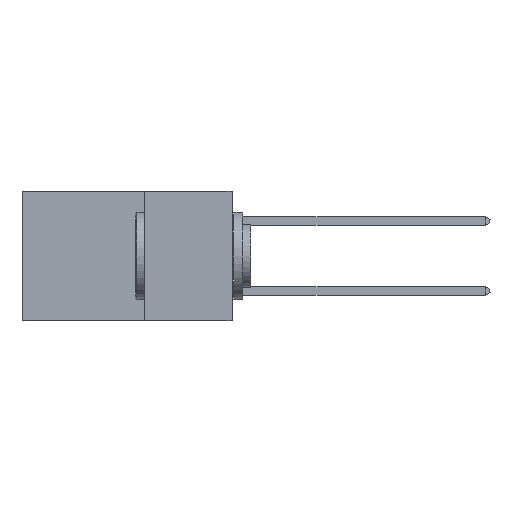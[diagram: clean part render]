
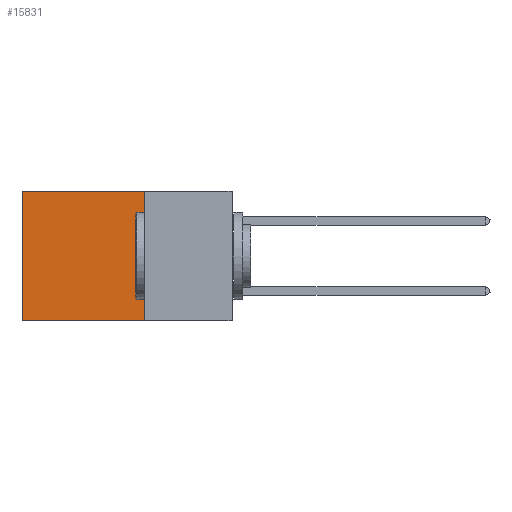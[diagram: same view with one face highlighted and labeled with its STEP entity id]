
A CAD part, left-side view. The second image highlights one B-rep face of the part: STEP entity #15831.
In plain terms, the highlighted planar face has unit normal (-1, 0, 0).
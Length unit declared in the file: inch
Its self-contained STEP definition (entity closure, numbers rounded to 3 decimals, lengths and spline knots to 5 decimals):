
#221 = EDGE_LOOP ( 'NONE', ( #6509, #34682, #23838, #32155 ) ) ;
#659 = VECTOR ( 'NONE', #8552, 39.37008 ) ;
#698 = EDGE_CURVE ( 'NONE', #30592, #21738, #38104, .T. ) ;
#722 = VECTOR ( 'NONE', #20256, 39.37008 ) ;
#741 = VERTEX_POINT ( 'NONE', #23607 ) ;
#1066 = VECTOR ( 'NONE', #27200, 39.37008 ) ;
#3652 = DIRECTION ( 'NONE',  ( 1., 0., 0. ) ) ;
#5477 = LINE ( 'NONE', #33560, #34969 ) ;
#6509 = ORIENTED_EDGE ( 'NONE', *, *, #698, .T. ) ;
#8521 = LINE ( 'NONE', #29310, #659 ) ;
#8552 = DIRECTION ( 'NONE',  ( 0., 0., -1. ) ) ;
#9136 = CARTESIAN_POINT ( 'NONE',  ( 0.2875, 0.25, 0. ) ) ;
#10933 = EDGE_CURVE ( 'NONE', #741, #38155, #8521, .T. ) ;
#11658 = EDGE_CURVE ( 'NONE', #741, #30592, #11702, .T. ) ;
#11702 = LINE ( 'NONE', #9136, #1066 ) ;
#15831 = ADVANCED_FACE ( 'NONE', ( #21496 ), #27659, .F. ) ;
#17510 = AXIS2_PLACEMENT_3D ( 'NONE', #30095, #3652, #18354 ) ;
#18354 = DIRECTION ( 'NONE',  ( 0., 0., -1. ) ) ;
#20256 = DIRECTION ( 'NONE',  ( 0., 0., -1. ) ) ;
#21496 = FACE_OUTER_BOUND ( 'NONE', #221, .T. ) ;
#21562 = CARTESIAN_POINT ( 'NONE',  ( 0.2875, 0.6, 0. ) ) ;
#21738 = VERTEX_POINT ( 'NONE', #22517 ) ;
#22413 = DIRECTION ( 'NONE',  ( 0., 1., 0. ) ) ;
#22517 = CARTESIAN_POINT ( 'NONE',  ( 0.2875, 0.6, -0.37 ) ) ;
#23607 = CARTESIAN_POINT ( 'NONE',  ( 0.2875, 0.25, 0. ) ) ;
#23838 = ORIENTED_EDGE ( 'NONE', *, *, #10933, .F. ) ;
#27200 = DIRECTION ( 'NONE',  ( 0., 1., 0. ) ) ;
#27659 = PLANE ( 'NONE',  #17510 ) ;
#28557 = CARTESIAN_POINT ( 'NONE',  ( 0.2875, 0.25, -0.37 ) ) ;
#29310 = CARTESIAN_POINT ( 'NONE',  ( 0.2875, 0.25, 0. ) ) ;
#29574 = CARTESIAN_POINT ( 'NONE',  ( 0.2875, 0.6, 0. ) ) ;
#30095 = CARTESIAN_POINT ( 'NONE',  ( 0.2875, 0.25, 0. ) ) ;
#30174 = EDGE_CURVE ( 'NONE', #38155, #21738, #5477, .T. ) ;
#30592 = VERTEX_POINT ( 'NONE', #21562 ) ;
#32155 = ORIENTED_EDGE ( 'NONE', *, *, #11658, .T. ) ;
#33560 = CARTESIAN_POINT ( 'NONE',  ( 0.2875, 0.25, -0.37 ) ) ;
#34682 = ORIENTED_EDGE ( 'NONE', *, *, #30174, .F. ) ;
#34969 = VECTOR ( 'NONE', #22413, 39.37008 ) ;
#38104 = LINE ( 'NONE', #29574, #722 ) ;
#38155 = VERTEX_POINT ( 'NONE', #28557 ) ;
